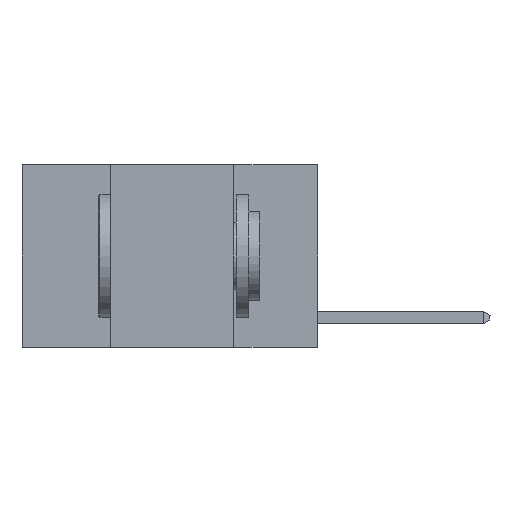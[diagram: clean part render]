
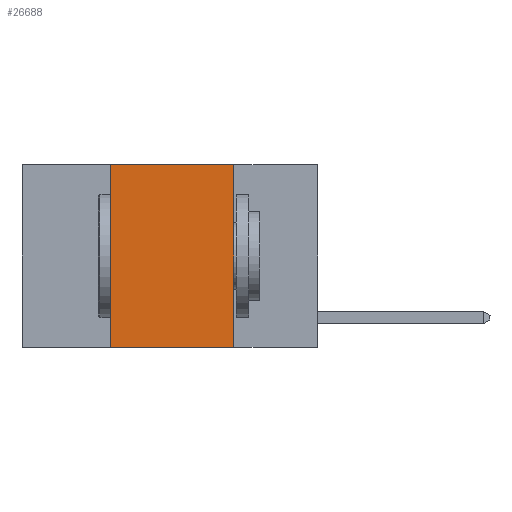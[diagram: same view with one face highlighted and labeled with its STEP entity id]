
A CAD part, left-side view. The second image highlights one B-rep face of the part: STEP entity #26688.
In plain terms, the highlighted planar face has unit normal (-1, 0, 0).
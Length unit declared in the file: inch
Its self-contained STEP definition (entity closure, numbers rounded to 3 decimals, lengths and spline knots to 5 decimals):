
#1317 = VECTOR ( 'NONE', #12560, 39.37008 ) ;
#2337 = VERTEX_POINT ( 'NONE', #18808 ) ;
#4108 = VERTEX_POINT ( 'NONE', #28311 ) ;
#5043 = AXIS2_PLACEMENT_3D ( 'NONE', #13925, #5279, #27293 ) ;
#5279 = DIRECTION ( 'NONE',  ( 1., 0., 0. ) ) ;
#6595 = VERTEX_POINT ( 'NONE', #20856 ) ;
#6723 = ORIENTED_EDGE ( 'NONE', *, *, #9281, .F. ) ;
#7121 = EDGE_CURVE ( 'NONE', #4108, #28411, #10128, .T. ) ;
#7241 = DIRECTION ( 'NONE',  ( 0., -1., 0. ) ) ;
#7634 = EDGE_CURVE ( 'NONE', #6595, #2337, #24069, .T. ) ;
#8299 = VECTOR ( 'NONE', #7241, 39.37008 ) ;
#9281 = EDGE_CURVE ( 'NONE', #28411, #6595, #11777, .T. ) ;
#9874 = EDGE_LOOP ( 'NONE', ( #18751, #6723, #28196, #23764 ) ) ;
#10128 = LINE ( 'NONE', #11173, #11858 ) ;
#10518 = FACE_OUTER_BOUND ( 'NONE', #9874, .T. ) ;
#10583 = CARTESIAN_POINT ( 'NONE',  ( 0., 0.17, 0. ) ) ;
#11173 = CARTESIAN_POINT ( 'NONE',  ( 0., 0.42, 0. ) ) ;
#11777 = LINE ( 'NONE', #20587, #8299 ) ;
#11858 = VECTOR ( 'NONE', #17914, 39.37008 ) ;
#12560 = DIRECTION ( 'NONE',  ( 0., -1., 0. ) ) ;
#13925 = CARTESIAN_POINT ( 'NONE',  ( 0., 0.6, 0. ) ) ;
#13929 = VECTOR ( 'NONE', #17211, 39.37008 ) ;
#13986 = CARTESIAN_POINT ( 'NONE',  ( 0., 0.42, 0. ) ) ;
#17116 = EDGE_CURVE ( 'NONE', #4108, #2337, #17660, .T. ) ;
#17211 = DIRECTION ( 'NONE',  ( 0., 0., -1. ) ) ;
#17660 = LINE ( 'NONE', #25546, #1317 ) ;
#17914 = DIRECTION ( 'NONE',  ( 0., 0., 1. ) ) ;
#18751 = ORIENTED_EDGE ( 'NONE', *, *, #7634, .F. ) ;
#18808 = CARTESIAN_POINT ( 'NONE',  ( 0., 0.17, -0.37 ) ) ;
#20587 = CARTESIAN_POINT ( 'NONE',  ( 0., 0.6, 0. ) ) ;
#20856 = CARTESIAN_POINT ( 'NONE',  ( 0., 0.17, 0. ) ) ;
#23764 = ORIENTED_EDGE ( 'NONE', *, *, #17116, .T. ) ;
#24069 = LINE ( 'NONE', #10583, #13929 ) ;
#25546 = CARTESIAN_POINT ( 'NONE',  ( 0., 0.6, -0.37 ) ) ;
#26688 = ADVANCED_FACE ( 'NONE', ( #10518 ), #27380, .F. ) ;
#27293 = DIRECTION ( 'NONE',  ( 0., 0., -1. ) ) ;
#27380 = PLANE ( 'NONE',  #5043 ) ;
#28196 = ORIENTED_EDGE ( 'NONE', *, *, #7121, .F. ) ;
#28311 = CARTESIAN_POINT ( 'NONE',  ( 0., 0.42, -0.37 ) ) ;
#28411 = VERTEX_POINT ( 'NONE', #13986 ) ;
